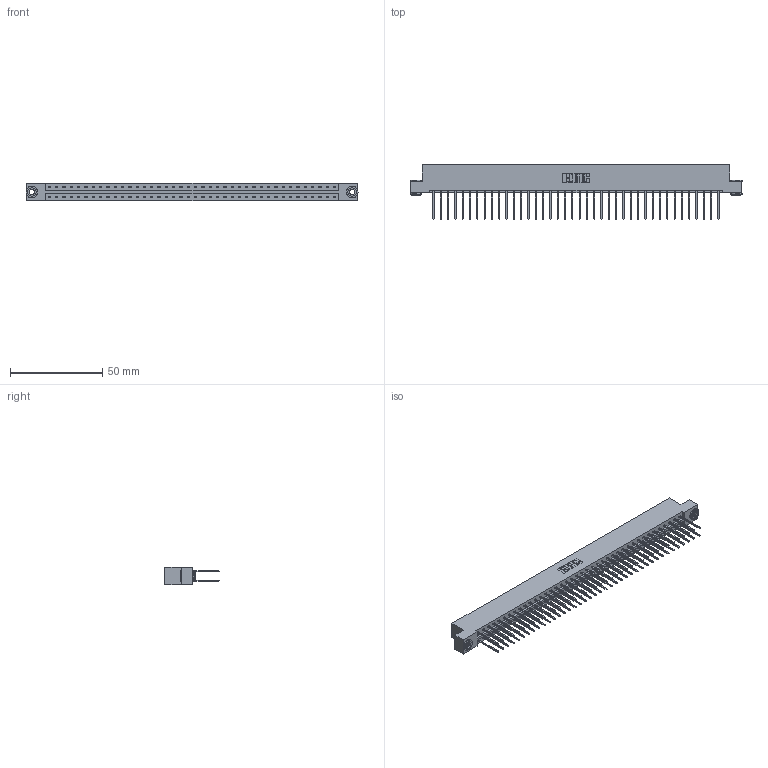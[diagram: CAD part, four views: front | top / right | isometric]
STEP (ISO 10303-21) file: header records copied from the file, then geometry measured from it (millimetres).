
FILE_DESCRIPTION (( 'STEP AP203' ), '1' );
FILE_NAME ('833-080-540-203.STEP', '2020-06-05T21:43:40', ( '' ), ( '' ), 'SwSTEP 2.0', 'SolidWorks 2020', '' );
FILE_SCHEMA (( 'CONFIG_CONTROL_DESIGN' ));
Length unit declared in the file: inch
Products named in the file (4): 833-080-540-203; 833 Part_Flush - .156 Dia - TH; 345-292-001_345-293-140; 345-250-002_345-250-002-102
Assembly tree (83 placements, depth 2):
  833-080-540-203
    833 Part_Flush - .156 Dia - TH
    345-292-001_345-293-140  x80
    345-250-002_345-250-002-102  x2
Bounding box: 180.04 x 29.47 x 9.4 mm (x, y, z)
Volume: 18684.5 mm3; surface area: 23778 mm2
Topology: 83 solids, 83 shells, 4312 faces, 12787 edges, 8414 vertices
Faces by surface type: plane 2960, cylinder 1344, cone 8
Entity records: 26660 total; most frequent: CARTESIAN_POINT 4397, ORIENTED_EDGE 4326, DIRECTION 3793, EDGE_CURVE 2163, LINE 2011, VECTOR 2011, VERTEX_POINT 1438, AXIS2_PLACEMENT_3D 891
